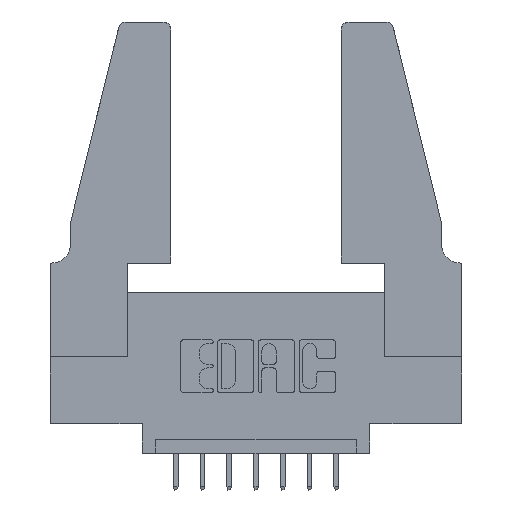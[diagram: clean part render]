
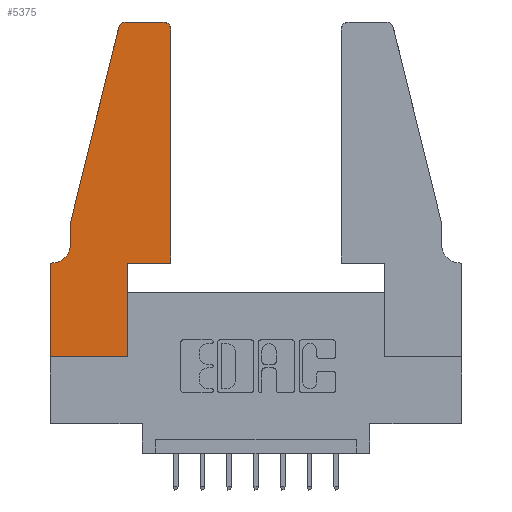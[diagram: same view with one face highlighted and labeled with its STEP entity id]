
A CAD part, top view. The second image highlights one B-rep face of the part: STEP entity #5375.
In plain terms, the highlighted planar face has unit normal (0, 0, 1).
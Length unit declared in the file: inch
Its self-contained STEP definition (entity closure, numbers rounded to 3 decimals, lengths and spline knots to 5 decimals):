
#29 = CARTESIAN_POINT ( 'NONE',  ( 0.0755, 0.5, 0.37 ) ) ;
#100 = LINE ( 'NONE', #8490, #1038 ) ;
#192 = DIRECTION ( 'NONE',  ( 1., 0., 0. ) ) ;
#228 = CARTESIAN_POINT ( 'NONE',  ( 0., 0.35, 0.37 ) ) ;
#377 = CARTESIAN_POINT ( 'NONE',  ( 0.4205, 1.22, 0.37 ) ) ;
#414 = PLANE ( 'NONE',  #5498 ) ;
#440 = VERTEX_POINT ( 'NONE', #11808 ) ;
#496 = EDGE_CURVE ( 'NONE', #11263, #3784, #4940, .T. ) ;
#508 = VECTOR ( 'NONE', #669, 39.37008 ) ;
#669 = DIRECTION ( 'NONE',  ( 1., 0., 0. ) ) ;
#1027 = CARTESIAN_POINT ( 'NONE',  ( 0.4505, 1.22, 0.37 ) ) ;
#1038 = VECTOR ( 'NONE', #5600, 39.37008 ) ;
#1273 = CARTESIAN_POINT ( 'NONE',  ( 0.4205, 1.25, 0.37 ) ) ;
#1334 = CARTESIAN_POINT ( 'NONE',  ( 0., 0.35, 0.37 ) ) ;
#1416 = DIRECTION ( 'NONE',  ( 1., 0., 0. ) ) ;
#1469 = VECTOR ( 'NONE', #3938, 39.37008 ) ;
#1882 = DIRECTION ( 'NONE',  ( -1., 0., 0. ) ) ;
#2347 = LINE ( 'NONE', #11609, #12087 ) ;
#2549 = LINE ( 'NONE', #10176, #508 ) ;
#2604 = CARTESIAN_POINT ( 'NONE',  ( 0.2605, 1.25, 0.37 ) ) ;
#2694 = AXIS2_PLACEMENT_3D ( 'NONE', #6176, #7179, #3092 ) ;
#2860 = CARTESIAN_POINT ( 'NONE',  ( 0.0755, 0.5, 0.37 ) ) ;
#2879 = EDGE_CURVE ( 'NONE', #7138, #4649, #3061, .T. ) ;
#2937 = EDGE_CURVE ( 'NONE', #10002, #4856, #6148, .T. ) ;
#2939 = LINE ( 'NONE', #2860, #9702 ) ;
#3061 = LINE ( 'NONE', #9496, #1469 ) ;
#3092 = DIRECTION ( 'NONE',  ( -1., 0., 0. ) ) ;
#3103 = FACE_OUTER_BOUND ( 'NONE', #10274, .T. ) ;
#3712 = CIRCLE ( 'NONE', #2694, 0.07 ) ;
#3784 = VERTEX_POINT ( 'NONE', #1273 ) ;
#3938 = DIRECTION ( 'NONE',  ( 0., -1., 0. ) ) ;
#4048 = CARTESIAN_POINT ( 'NONE',  ( 0.4505, 0.35, 0.37 ) ) ;
#4093 = VECTOR ( 'NONE', #1882, 39.37008 ) ;
#4122 = EDGE_CURVE ( 'NONE', #440, #7138, #11450, .T. ) ;
#4149 = CARTESIAN_POINT ( 'NONE',  ( 0.2865, 0., 0.37 ) ) ;
#4274 = CARTESIAN_POINT ( 'NONE',  ( 0.2865, 0.35, 0.37 ) ) ;
#4578 = CARTESIAN_POINT ( 'NONE',  ( 0.25487, 1.22718, 0.37 ) ) ;
#4649 = VERTEX_POINT ( 'NONE', #12069 ) ;
#4737 = EDGE_CURVE ( 'NONE', #3784, #11487, #5369, .T. ) ;
#4856 = VERTEX_POINT ( 'NONE', #10359 ) ;
#4931 = DIRECTION ( 'NONE',  ( 0., 1., 0. ) ) ;
#4940 = CIRCLE ( 'NONE', #6158, 0.03 ) ;
#5086 = EDGE_CURVE ( 'NONE', #5828, #8943, #2347, .T. ) ;
#5160 = EDGE_CURVE ( 'NONE', #11487, #7395, #7106, .T. ) ;
#5275 = LINE ( 'NONE', #4048, #8103 ) ;
#5297 = DIRECTION ( 'NONE',  ( 0., 0., 1. ) ) ;
#5369 = LINE ( 'NONE', #2604, #6499 ) ;
#5375 = ADVANCED_FACE ( 'NONE', ( #3103 ), #414, .T. ) ;
#5498 = AXIS2_PLACEMENT_3D ( 'NONE', #228, #5922, #7851 ) ;
#5600 = DIRECTION ( 'NONE',  ( 0., 1., 0. ) ) ;
#5775 = CARTESIAN_POINT ( 'NONE',  ( 0.0755, 0.35, 0.37 ) ) ;
#5828 = VERTEX_POINT ( 'NONE', #4149 ) ;
#5922 = DIRECTION ( 'NONE',  ( 0., 0., 1. ) ) ;
#6069 = DIRECTION ( 'NONE',  ( 0., -1., 0. ) ) ;
#6148 = LINE ( 'NONE', #10048, #12269 ) ;
#6158 = AXIS2_PLACEMENT_3D ( 'NONE', #377, #6331, #9461 ) ;
#6176 = CARTESIAN_POINT ( 'NONE',  ( 0.0055, 0.42, 0.37 ) ) ;
#6331 = DIRECTION ( 'NONE',  ( 0., 0., 1. ) ) ;
#6398 = DIRECTION ( 'NONE',  ( -1., 0., 0. ) ) ;
#6499 = VECTOR ( 'NONE', #6398, 39.37008 ) ;
#6503 = CARTESIAN_POINT ( 'NONE',  ( 0.284, 1.22, 0.37 ) ) ;
#6507 = AXIS2_PLACEMENT_3D ( 'NONE', #6503, #5297, #1416 ) ;
#6511 = EDGE_CURVE ( 'NONE', #8651, #11263, #100, .T. ) ;
#7106 = CIRCLE ( 'NONE', #6507, 0.03 ) ;
#7138 = VERTEX_POINT ( 'NONE', #1334 ) ;
#7179 = DIRECTION ( 'NONE',  ( 0., 0., -1. ) ) ;
#7325 = ORIENTED_EDGE ( 'NONE', *, *, #8919, .T. ) ;
#7395 = VERTEX_POINT ( 'NONE', #4578 ) ;
#7415 = ORIENTED_EDGE ( 'NONE', *, *, #8391, .T. ) ;
#7633 = DIRECTION ( 'NONE',  ( -0.239, -0.971, 0. ) ) ;
#7827 = ORIENTED_EDGE ( 'NONE', *, *, #2937, .T. ) ;
#7851 = DIRECTION ( 'NONE',  ( 1., 0., 0. ) ) ;
#8103 = VECTOR ( 'NONE', #192, 39.37008 ) ;
#8391 = EDGE_CURVE ( 'NONE', #4649, #5828, #2549, .T. ) ;
#8490 = CARTESIAN_POINT ( 'NONE',  ( 0.4505, 0.35, 0.37 ) ) ;
#8651 = VERTEX_POINT ( 'NONE', #9719 ) ;
#8762 = ORIENTED_EDGE ( 'NONE', *, *, #4737, .T. ) ;
#8910 = ORIENTED_EDGE ( 'NONE', *, *, #496, .T. ) ;
#8919 = EDGE_CURVE ( 'NONE', #4856, #440, #3712, .T. ) ;
#8943 = VERTEX_POINT ( 'NONE', #4274 ) ;
#9047 = EDGE_CURVE ( 'NONE', #8943, #8651, #5275, .T. ) ;
#9160 = CARTESIAN_POINT ( 'NONE',  ( 0.284, 1.25, 0.37 ) ) ;
#9461 = DIRECTION ( 'NONE',  ( 1., 0., 0. ) ) ;
#9496 = CARTESIAN_POINT ( 'NONE',  ( 0., 0., 0.37 ) ) ;
#9702 = VECTOR ( 'NONE', #7633, 39.37008 ) ;
#9719 = CARTESIAN_POINT ( 'NONE',  ( 0.4505, 0.35, 0.37 ) ) ;
#9731 = ORIENTED_EDGE ( 'NONE', *, *, #6511, .T. ) ;
#10002 = VERTEX_POINT ( 'NONE', #29 ) ;
#10048 = CARTESIAN_POINT ( 'NONE',  ( 0.0755, 0.5, 0.37 ) ) ;
#10176 = CARTESIAN_POINT ( 'NONE',  ( 0., 0., 0.37 ) ) ;
#10274 = EDGE_LOOP ( 'NONE', ( #8762, #11157, #11398, #7827, #7325, #11236, #10707, #7415, #10722, #11824, #9731, #8910 ) ) ;
#10359 = CARTESIAN_POINT ( 'NONE',  ( 0.0755, 0.42, 0.37 ) ) ;
#10707 = ORIENTED_EDGE ( 'NONE', *, *, #2879, .T. ) ;
#10722 = ORIENTED_EDGE ( 'NONE', *, *, #5086, .T. ) ;
#10871 = EDGE_CURVE ( 'NONE', #7395, #10002, #2939, .T. ) ;
#11157 = ORIENTED_EDGE ( 'NONE', *, *, #5160, .T. ) ;
#11236 = ORIENTED_EDGE ( 'NONE', *, *, #4122, .T. ) ;
#11263 = VERTEX_POINT ( 'NONE', #1027 ) ;
#11398 = ORIENTED_EDGE ( 'NONE', *, *, #10871, .T. ) ;
#11450 = LINE ( 'NONE', #5775, #4093 ) ;
#11487 = VERTEX_POINT ( 'NONE', #9160 ) ;
#11609 = CARTESIAN_POINT ( 'NONE',  ( 0.2865, 0.35, 0.37 ) ) ;
#11808 = CARTESIAN_POINT ( 'NONE',  ( 0.0055, 0.35, 0.37 ) ) ;
#11824 = ORIENTED_EDGE ( 'NONE', *, *, #9047, .T. ) ;
#12069 = CARTESIAN_POINT ( 'NONE',  ( 0., 0., 0.37 ) ) ;
#12087 = VECTOR ( 'NONE', #4931, 39.37008 ) ;
#12269 = VECTOR ( 'NONE', #6069, 39.37008 ) ;
